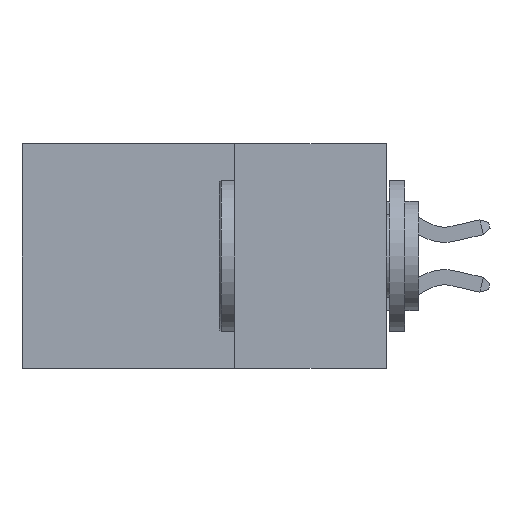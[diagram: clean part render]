
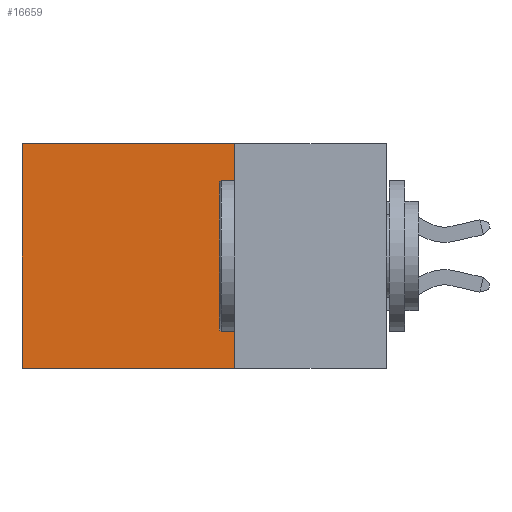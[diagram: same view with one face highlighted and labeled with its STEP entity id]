
A CAD part, left-side view. The second image highlights one B-rep face of the part: STEP entity #16659.
In plain terms, the highlighted planar face has unit normal (-1, 0, 0).
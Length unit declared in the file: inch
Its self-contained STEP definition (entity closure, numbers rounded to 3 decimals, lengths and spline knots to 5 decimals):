
#102 = VERTEX_POINT ( 'NONE', #14148 ) ;
#137 = VERTEX_POINT ( 'NONE', #4107 ) ;
#164 = PLANE ( 'NONE',  #19574 ) ;
#447 = ORIENTED_EDGE ( 'NONE', *, *, #19964, .T. ) ;
#1187 = DIRECTION ( 'NONE',  ( 0., 0., -1. ) ) ;
#1670 = CARTESIAN_POINT ( 'NONE',  ( 0.2615, 0.6, -0.37 ) ) ;
#2085 = CARTESIAN_POINT ( 'NONE',  ( 0.2615, 0.25, 0. ) ) ;
#2105 = CARTESIAN_POINT ( 'NONE',  ( 0.2615, 0.6, -0.37 ) ) ;
#2623 = VECTOR ( 'NONE', #3657, 39.37008 ) ;
#3322 = CARTESIAN_POINT ( 'NONE',  ( 0.2615, 0.25, -0.37 ) ) ;
#3551 = DIRECTION ( 'NONE',  ( 0., 0., -1. ) ) ;
#3657 = DIRECTION ( 'NONE',  ( 0., 1., 0. ) ) ;
#3661 = CARTESIAN_POINT ( 'NONE',  ( 0.2615, 0.25, -0.37 ) ) ;
#3770 = DIRECTION ( 'NONE',  ( 0., 1., 0. ) ) ;
#4107 = CARTESIAN_POINT ( 'NONE',  ( 0.2615, 0.25, 0. ) ) ;
#6123 = VECTOR ( 'NONE', #3770, 39.37008 ) ;
#6955 = LINE ( 'NONE', #1670, #21224 ) ;
#7198 = EDGE_LOOP ( 'NONE', ( #447, #10040, #16586, #8327 ) ) ;
#7350 = EDGE_CURVE ( 'NONE', #137, #16657, #21814, .T. ) ;
#8327 = ORIENTED_EDGE ( 'NONE', *, *, #10009, .T. ) ;
#9864 = EDGE_CURVE ( 'NONE', #16657, #11321, #19120, .T. ) ;
#10009 = EDGE_CURVE ( 'NONE', #137, #102, #14367, .T. ) ;
#10040 = ORIENTED_EDGE ( 'NONE', *, *, #9864, .F. ) ;
#11321 = VERTEX_POINT ( 'NONE', #2105 ) ;
#13907 = CARTESIAN_POINT ( 'NONE',  ( 0.2615, 0.25, -0.37 ) ) ;
#14148 = CARTESIAN_POINT ( 'NONE',  ( 0.2615, 0.6, 0. ) ) ;
#14367 = LINE ( 'NONE', #2085, #6123 ) ;
#15054 = CARTESIAN_POINT ( 'NONE',  ( 0.2615, 0.25, -0.37 ) ) ;
#16586 = ORIENTED_EDGE ( 'NONE', *, *, #7350, .F. ) ;
#16657 = VERTEX_POINT ( 'NONE', #3661 ) ;
#16659 = ADVANCED_FACE ( 'NONE', ( #19011 ), #164, .F. ) ;
#19011 = FACE_OUTER_BOUND ( 'NONE', #7198, .T. ) ;
#19120 = LINE ( 'NONE', #3322, #2623 ) ;
#19360 = VECTOR ( 'NONE', #1187, 39.37008 ) ;
#19574 = AXIS2_PLACEMENT_3D ( 'NONE', #13907, #20805, #3551 ) ;
#19964 = EDGE_CURVE ( 'NONE', #102, #11321, #6955, .T. ) ;
#20620 = DIRECTION ( 'NONE',  ( 0., 0., -1. ) ) ;
#20805 = DIRECTION ( 'NONE',  ( 1., 0., 0. ) ) ;
#21224 = VECTOR ( 'NONE', #20620, 39.37008 ) ;
#21814 = LINE ( 'NONE', #15054, #19360 ) ;
